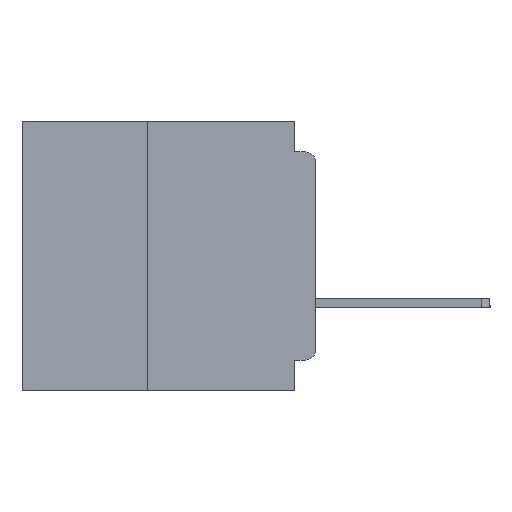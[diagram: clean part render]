
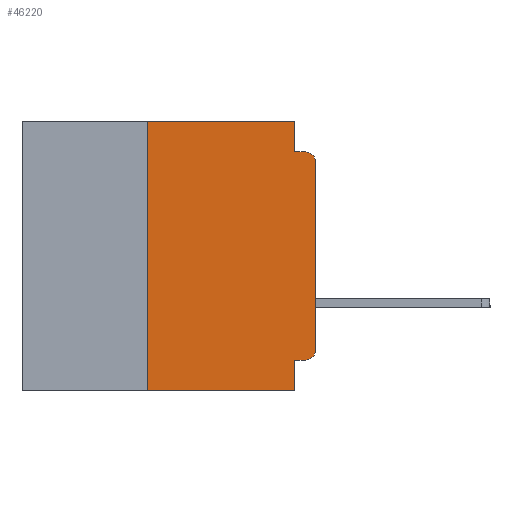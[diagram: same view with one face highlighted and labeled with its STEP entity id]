
A CAD part, left-side view. The second image highlights one B-rep face of the part: STEP entity #46220.
In plain terms, the highlighted planar face has unit normal (-1, 0, 0).
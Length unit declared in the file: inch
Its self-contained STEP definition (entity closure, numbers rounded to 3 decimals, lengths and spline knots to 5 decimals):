
#1845 = VECTOR ( 'NONE', #62515, 39.37008 ) ;
#1930 = VERTEX_POINT ( 'NONE', #28895 ) ;
#2067 = CARTESIAN_POINT ( 'NONE',  ( 0., 0.25, -0.4 ) ) ;
#3364 = CARTESIAN_POINT ( 'NONE',  ( 0., 0.015, -0.355 ) ) ;
#4097 = VECTOR ( 'NONE', #59843, 39.37008 ) ;
#4595 = EDGE_CURVE ( 'NONE', #29969, #17509, #6803, .T. ) ;
#4751 = DIRECTION ( 'NONE',  ( 0., 0., -1. ) ) ;
#5041 = DIRECTION ( 'NONE',  ( 0., 0., -1. ) ) ;
#5239 = VECTOR ( 'NONE', #13861, 39.37008 ) ;
#5443 = PLANE ( 'NONE',  #44066 ) ;
#5490 = DIRECTION ( 'NONE',  ( 0., -1., 0. ) ) ;
#5609 = ORIENTED_EDGE ( 'NONE', *, *, #4595, .F. ) ;
#5737 = ORIENTED_EDGE ( 'NONE', *, *, #31526, .F. ) ;
#6079 = VECTOR ( 'NONE', #5041, 39.37008 ) ;
#6803 = LINE ( 'NONE', #14001, #5239 ) ;
#7980 = CARTESIAN_POINT ( 'NONE',  ( 0., 0.031, -0.355 ) ) ;
#8656 = VECTOR ( 'NONE', #36777, 39.37008 ) ;
#8937 = VERTEX_POINT ( 'NONE', #33020 ) ;
#9055 = CARTESIAN_POINT ( 'NONE',  ( 0., 0.031, -0.4 ) ) ;
#9184 = VECTOR ( 'NONE', #34593, 39.37008 ) ;
#10396 = EDGE_CURVE ( 'NONE', #23543, #29969, #48189, .T. ) ;
#11840 = LINE ( 'NONE', #63446, #26361 ) ;
#11964 = ORIENTED_EDGE ( 'NONE', *, *, #10396, .F. ) ;
#13861 = DIRECTION ( 'NONE',  ( 0., -1., 0. ) ) ;
#14001 = CARTESIAN_POINT ( 'NONE',  ( 0., 0., -0.045 ) ) ;
#15156 = CARTESIAN_POINT ( 'NONE',  ( 0., 0.031, 0. ) ) ;
#16133 = LINE ( 'NONE', #34447, #6079 ) ;
#17239 = LINE ( 'NONE', #25725, #4097 ) ;
#17497 = VERTEX_POINT ( 'NONE', #7980 ) ;
#17509 = VERTEX_POINT ( 'NONE', #61789 ) ;
#20241 = VERTEX_POINT ( 'NONE', #9055 ) ;
#20285 = DIRECTION ( 'NONE',  ( 1., 0., 0. ) ) ;
#20977 = DIRECTION ( 'NONE',  ( -1., 0., 0. ) ) ;
#23387 = AXIS2_PLACEMENT_3D ( 'NONE', #50210, #20977, #55096 ) ;
#23543 = VERTEX_POINT ( 'NONE', #52460 ) ;
#23623 = CIRCLE ( 'NONE', #23387, 0.015 ) ;
#24190 = EDGE_LOOP ( 'NONE', ( #44658, #42818, #5609, #11964, #57133, #5737, #34079, #60825, #45682, #59201 ) ) ;
#25557 = CARTESIAN_POINT ( 'NONE',  ( 0., 0.031, -0.045 ) ) ;
#25725 = CARTESIAN_POINT ( 'NONE',  ( 0., 0.437, 0. ) ) ;
#26361 = VECTOR ( 'NONE', #39173, 39.37008 ) ;
#28895 = CARTESIAN_POINT ( 'NONE',  ( 0., 0., -0.06 ) ) ;
#29801 = EDGE_CURVE ( 'NONE', #45428, #8937, #42805, .T. ) ;
#29969 = VERTEX_POINT ( 'NONE', #25557 ) ;
#31526 = EDGE_CURVE ( 'NONE', #32193, #36626, #42557, .T. ) ;
#31909 = CARTESIAN_POINT ( 'NONE',  ( 0., 0., -0.355 ) ) ;
#32107 = EDGE_CURVE ( 'NONE', #36626, #23543, #17239, .T. ) ;
#32193 = VERTEX_POINT ( 'NONE', #2067 ) ;
#32409 = EDGE_CURVE ( 'NONE', #8937, #1930, #11840, .T. ) ;
#32707 = FACE_OUTER_BOUND ( 'NONE', #24190, .T. ) ;
#33020 = CARTESIAN_POINT ( 'NONE',  ( 0., 0., -0.34 ) ) ;
#34079 = ORIENTED_EDGE ( 'NONE', *, *, #55739, .T. ) ;
#34165 = DIRECTION ( 'NONE',  ( -1., 0., 0. ) ) ;
#34447 = CARTESIAN_POINT ( 'NONE',  ( 0., 0.031, -0.4 ) ) ;
#34593 = DIRECTION ( 'NONE',  ( 0., 0., -1. ) ) ;
#34705 = LINE ( 'NONE', #31909, #8656 ) ;
#36626 = VERTEX_POINT ( 'NONE', #49672 ) ;
#36777 = DIRECTION ( 'NONE',  ( 0., 1., 0. ) ) ;
#39173 = DIRECTION ( 'NONE',  ( 0., 0., 1. ) ) ;
#39571 = CARTESIAN_POINT ( 'NONE',  ( 0., 0.437, -0.4 ) ) ;
#42557 = LINE ( 'NONE', #42943, #1845 ) ;
#42805 = CIRCLE ( 'NONE', #50501, 0.015 ) ;
#42818 = ORIENTED_EDGE ( 'NONE', *, *, #53502, .T. ) ;
#42943 = CARTESIAN_POINT ( 'NONE',  ( 0., 0.25, -0.4 ) ) ;
#43822 = EDGE_CURVE ( 'NONE', #17497, #20241, #16133, .T. ) ;
#44066 = AXIS2_PLACEMENT_3D ( 'NONE', #49509, #20285, #54404 ) ;
#44080 = VECTOR ( 'NONE', #5490, 39.37008 ) ;
#44658 = ORIENTED_EDGE ( 'NONE', *, *, #32409, .T. ) ;
#45428 = VERTEX_POINT ( 'NONE', #3364 ) ;
#45682 = ORIENTED_EDGE ( 'NONE', *, *, #57184, .F. ) ;
#46220 = ADVANCED_FACE ( 'NONE', ( #32707 ), #5443, .F. ) ;
#48189 = LINE ( 'NONE', #15156, #9184 ) ;
#49509 = CARTESIAN_POINT ( 'NONE',  ( 0., 0.437, 0. ) ) ;
#49672 = CARTESIAN_POINT ( 'NONE',  ( 0., 0.25, 0. ) ) ;
#50210 = CARTESIAN_POINT ( 'NONE',  ( 0., 0.015, -0.06 ) ) ;
#50501 = AXIS2_PLACEMENT_3D ( 'NONE', #63331, #34165, #4751 ) ;
#52460 = CARTESIAN_POINT ( 'NONE',  ( 0., 0.031, 0. ) ) ;
#53502 = EDGE_CURVE ( 'NONE', #1930, #17509, #23623, .T. ) ;
#54404 = DIRECTION ( 'NONE',  ( 0., 0., -1. ) ) ;
#55096 = DIRECTION ( 'NONE',  ( 0., 0., -1. ) ) ;
#55739 = EDGE_CURVE ( 'NONE', #32193, #20241, #57006, .T. ) ;
#57006 = LINE ( 'NONE', #39571, #44080 ) ;
#57133 = ORIENTED_EDGE ( 'NONE', *, *, #32107, .F. ) ;
#57184 = EDGE_CURVE ( 'NONE', #45428, #17497, #34705, .T. ) ;
#59201 = ORIENTED_EDGE ( 'NONE', *, *, #29801, .T. ) ;
#59843 = DIRECTION ( 'NONE',  ( 0., -1., 0. ) ) ;
#60825 = ORIENTED_EDGE ( 'NONE', *, *, #43822, .F. ) ;
#61789 = CARTESIAN_POINT ( 'NONE',  ( 0., 0.015, -0.045 ) ) ;
#62515 = DIRECTION ( 'NONE',  ( 0., 0., 1. ) ) ;
#63331 = CARTESIAN_POINT ( 'NONE',  ( 0., 0.015, -0.34 ) ) ;
#63446 = CARTESIAN_POINT ( 'NONE',  ( 0., 0., 0. ) ) ;
